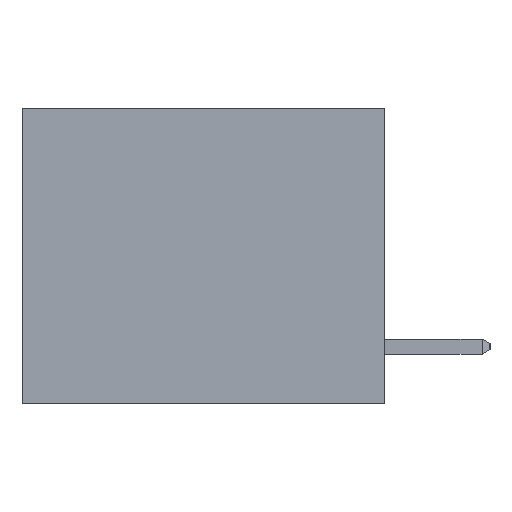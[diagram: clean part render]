
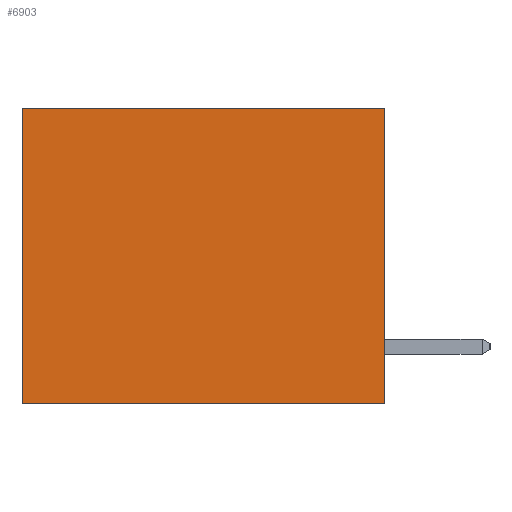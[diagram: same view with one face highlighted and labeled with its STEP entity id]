
A CAD part, left-side view. The second image highlights one B-rep face of the part: STEP entity #6903.
In plain terms, the highlighted planar face has unit normal (-1, 0, 0).
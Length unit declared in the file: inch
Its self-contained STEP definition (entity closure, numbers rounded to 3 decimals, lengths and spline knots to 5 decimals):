
#806 = EDGE_CURVE ( 'NONE', #14190, #14126, #13519, .T. ) ;
#1300 = ORIENTED_EDGE ( 'NONE', *, *, #3026, .T. ) ;
#1873 = DIRECTION ( 'NONE',  ( 0., 0., -1. ) ) ;
#1913 = VECTOR ( 'NONE', #15967, 39.37008 ) ;
#2145 = CARTESIAN_POINT ( 'NONE',  ( 0.3165, 0., -0.49 ) ) ;
#2373 = ORIENTED_EDGE ( 'NONE', *, *, #806, .T. ) ;
#2481 = CARTESIAN_POINT ( 'NONE',  ( 0.3165, 0., -0.49 ) ) ;
#3026 = EDGE_CURVE ( 'NONE', #14126, #12124, #4547, .T. ) ;
#3368 = AXIS2_PLACEMENT_3D ( 'NONE', #2145, #7236, #7168 ) ;
#3987 = EDGE_CURVE ( 'NONE', #6988, #12124, #15137, .T. ) ;
#4547 = LINE ( 'NONE', #13477, #1913 ) ;
#6682 = EDGE_CURVE ( 'NONE', #14190, #6988, #14584, .T. ) ;
#6694 = EDGE_LOOP ( 'NONE', ( #1300, #13460, #16397, #2373 ) ) ;
#6903 = ADVANCED_FACE ( 'NONE', ( #7702 ), #15018, .F. ) ;
#6965 = CARTESIAN_POINT ( 'NONE',  ( 0.3165, 0.6, 0. ) ) ;
#6988 = VERTEX_POINT ( 'NONE', #2481 ) ;
#7023 = CARTESIAN_POINT ( 'NONE',  ( 0.3165, 0., -0.49 ) ) ;
#7168 = DIRECTION ( 'NONE',  ( 0., 0., -1. ) ) ;
#7236 = DIRECTION ( 'NONE',  ( 1., 0., 0. ) ) ;
#7488 = VECTOR ( 'NONE', #10809, 39.37008 ) ;
#7702 = FACE_OUTER_BOUND ( 'NONE', #6694, .T. ) ;
#8155 = CARTESIAN_POINT ( 'NONE',  ( 0.3165, 0., 0. ) ) ;
#8326 = VECTOR ( 'NONE', #1873, 39.37008 ) ;
#8334 = CARTESIAN_POINT ( 'NONE',  ( 0.3165, 0., -0.49 ) ) ;
#10340 = VECTOR ( 'NONE', #10768, 39.37008 ) ;
#10768 = DIRECTION ( 'NONE',  ( 0., 1., 0. ) ) ;
#10809 = DIRECTION ( 'NONE',  ( 0., 1., 0. ) ) ;
#12124 = VERTEX_POINT ( 'NONE', #16213 ) ;
#13460 = ORIENTED_EDGE ( 'NONE', *, *, #3987, .F. ) ;
#13477 = CARTESIAN_POINT ( 'NONE',  ( 0.3165, 0.6, -0.49 ) ) ;
#13519 = LINE ( 'NONE', #8155, #7488 ) ;
#13607 = CARTESIAN_POINT ( 'NONE',  ( 0.3165, 0., 0. ) ) ;
#14126 = VERTEX_POINT ( 'NONE', #6965 ) ;
#14190 = VERTEX_POINT ( 'NONE', #13607 ) ;
#14584 = LINE ( 'NONE', #7023, #8326 ) ;
#15018 = PLANE ( 'NONE',  #3368 ) ;
#15137 = LINE ( 'NONE', #8334, #10340 ) ;
#15967 = DIRECTION ( 'NONE',  ( 0., 0., -1. ) ) ;
#16213 = CARTESIAN_POINT ( 'NONE',  ( 0.3165, 0.6, -0.49 ) ) ;
#16397 = ORIENTED_EDGE ( 'NONE', *, *, #6682, .F. ) ;
